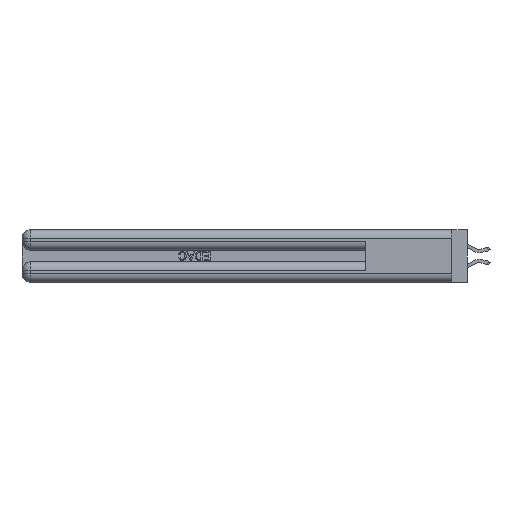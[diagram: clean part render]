
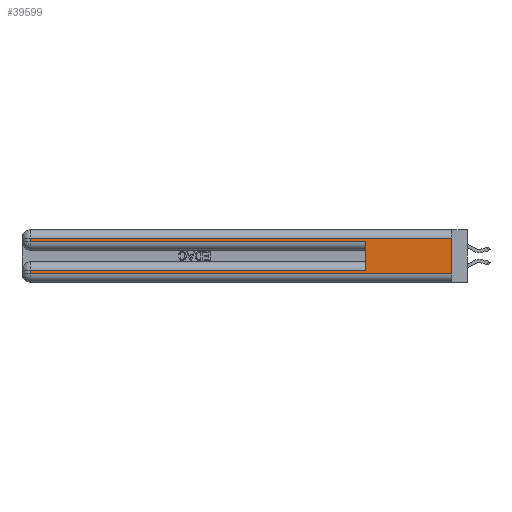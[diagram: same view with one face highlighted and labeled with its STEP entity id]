
A CAD part, left-side view. The second image highlights one B-rep face of the part: STEP entity #39599.
In plain terms, the highlighted planar face has unit normal (-1, 0, 0).
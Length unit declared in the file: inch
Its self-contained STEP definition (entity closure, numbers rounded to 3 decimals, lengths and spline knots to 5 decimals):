
#125 = LINE ( 'NONE', #30301, #16042 ) ;
#592 = AXIS2_PLACEMENT_3D ( 'NONE', #8390, #25172, #1173 ) ;
#846 = CARTESIAN_POINT ( 'NONE',  ( 0., 0., 0.06 ) ) ;
#1173 = DIRECTION ( 'NONE',  ( 0., 0., -1. ) ) ;
#2651 = LINE ( 'NONE', #26978, #21674 ) ;
#3010 = DIRECTION ( 'NONE',  ( 0., 1., 0. ) ) ;
#5015 = LINE ( 'NONE', #6456, #19834 ) ;
#5460 = VERTEX_POINT ( 'NONE', #28078 ) ;
#5599 = CARTESIAN_POINT ( 'NONE',  ( 0., 0.6, 0.085 ) ) ;
#5759 = EDGE_CURVE ( 'NONE', #13648, #21615, #8605, .T. ) ;
#5772 = CARTESIAN_POINT ( 'NONE',  ( 0., 0.6, 0.145 ) ) ;
#5888 = EDGE_CURVE ( 'NONE', #30704, #6565, #125, .T. ) ;
#6456 = CARTESIAN_POINT ( 'NONE',  ( 0., 2.94, 0.37 ) ) ;
#6565 = VERTEX_POINT ( 'NONE', #23242 ) ;
#6847 = CARTESIAN_POINT ( 'NONE',  ( 0., 0., 0.06 ) ) ;
#7299 = VECTOR ( 'NONE', #40492, 39.37008 ) ;
#8170 = EDGE_CURVE ( 'NONE', #13245, #15638, #13180, .T. ) ;
#8193 = CARTESIAN_POINT ( 'NONE',  ( 0., 2.94, 0.06 ) ) ;
#8288 = ORIENTED_EDGE ( 'NONE', *, *, #8170, .T. ) ;
#8390 = CARTESIAN_POINT ( 'NONE',  ( 0., 0., 0.37 ) ) ;
#8605 = LINE ( 'NONE', #5772, #29272 ) ;
#8921 = ORIENTED_EDGE ( 'NONE', *, *, #41086, .T. ) ;
#9336 = CARTESIAN_POINT ( 'NONE',  ( 0., 2.94, 0.31 ) ) ;
#9854 = DIRECTION ( 'NONE',  ( 0., 0., -1. ) ) ;
#10110 = ORIENTED_EDGE ( 'NONE', *, *, #5759, .F. ) ;
#12299 = DIRECTION ( 'NONE',  ( 0., 0., 1. ) ) ;
#12567 = CARTESIAN_POINT ( 'NONE',  ( 0., 0., 0.37 ) ) ;
#13180 = LINE ( 'NONE', #6847, #7299 ) ;
#13245 = VERTEX_POINT ( 'NONE', #8193 ) ;
#13648 = VERTEX_POINT ( 'NONE', #5599 ) ;
#15638 = VERTEX_POINT ( 'NONE', #846 ) ;
#15971 = DIRECTION ( 'NONE',  ( 0., 0., -1. ) ) ;
#16042 = VECTOR ( 'NONE', #43541, 39.37008 ) ;
#16485 = ORIENTED_EDGE ( 'NONE', *, *, #34179, .F. ) ;
#16754 = ORIENTED_EDGE ( 'NONE', *, *, #26532, .T. ) ;
#19834 = VECTOR ( 'NONE', #9854, 39.37008 ) ;
#19869 = EDGE_LOOP ( 'NONE', ( #16485, #36131, #25217, #8921, #10110, #39750, #16754, #8288 ) ) ;
#20080 = FACE_OUTER_BOUND ( 'NONE', #19869, .T. ) ;
#20148 = VERTEX_POINT ( 'NONE', #28037 ) ;
#20405 = EDGE_CURVE ( 'NONE', #5460, #30704, #2651, .T. ) ;
#21060 = VECTOR ( 'NONE', #29595, 39.37008 ) ;
#21615 = VERTEX_POINT ( 'NONE', #24046 ) ;
#21674 = VECTOR ( 'NONE', #42979, 39.37008 ) ;
#23234 = CARTESIAN_POINT ( 'NONE',  ( 0., 0., 0.085 ) ) ;
#23242 = CARTESIAN_POINT ( 'NONE',  ( 0., 2.94, 0.285 ) ) ;
#23381 = VECTOR ( 'NONE', #3010, 39.37008 ) ;
#24046 = CARTESIAN_POINT ( 'NONE',  ( 0., 0.6, 0.285 ) ) ;
#24177 = LINE ( 'NONE', #12567, #25289 ) ;
#25172 = DIRECTION ( 'NONE',  ( 1., 0., 0. ) ) ;
#25217 = ORIENTED_EDGE ( 'NONE', *, *, #5888, .T. ) ;
#25289 = VECTOR ( 'NONE', #15971, 39.37008 ) ;
#25507 = LINE ( 'NONE', #23234, #23381 ) ;
#26532 = EDGE_CURVE ( 'NONE', #20148, #13245, #5015, .T. ) ;
#26978 = CARTESIAN_POINT ( 'NONE',  ( 0., 0., 0.31 ) ) ;
#28037 = CARTESIAN_POINT ( 'NONE',  ( 0., 2.94, 0.085 ) ) ;
#28078 = CARTESIAN_POINT ( 'NONE',  ( 0., 0., 0.31 ) ) ;
#29272 = VECTOR ( 'NONE', #12299, 39.37008 ) ;
#29595 = DIRECTION ( 'NONE',  ( 0., -1., 0. ) ) ;
#30301 = CARTESIAN_POINT ( 'NONE',  ( 0., 2.94, 0.37 ) ) ;
#30704 = VERTEX_POINT ( 'NONE', #9336 ) ;
#33692 = EDGE_CURVE ( 'NONE', #13648, #20148, #25507, .T. ) ;
#34179 = EDGE_CURVE ( 'NONE', #5460, #15638, #24177, .T. ) ;
#35324 = PLANE ( 'NONE',  #592 ) ;
#36131 = ORIENTED_EDGE ( 'NONE', *, *, #20405, .T. ) ;
#39599 = ADVANCED_FACE ( 'NONE', ( #20080 ), #35324, .F. ) ;
#39750 = ORIENTED_EDGE ( 'NONE', *, *, #33692, .T. ) ;
#40492 = DIRECTION ( 'NONE',  ( 0., -1., 0. ) ) ;
#41086 = EDGE_CURVE ( 'NONE', #6565, #21615, #43254, .T. ) ;
#42979 = DIRECTION ( 'NONE',  ( 0., 1., 0. ) ) ;
#43254 = LINE ( 'NONE', #43274, #21060 ) ;
#43274 = CARTESIAN_POINT ( 'NONE',  ( 0., 0., 0.285 ) ) ;
#43541 = DIRECTION ( 'NONE',  ( 0., 0., -1. ) ) ;
